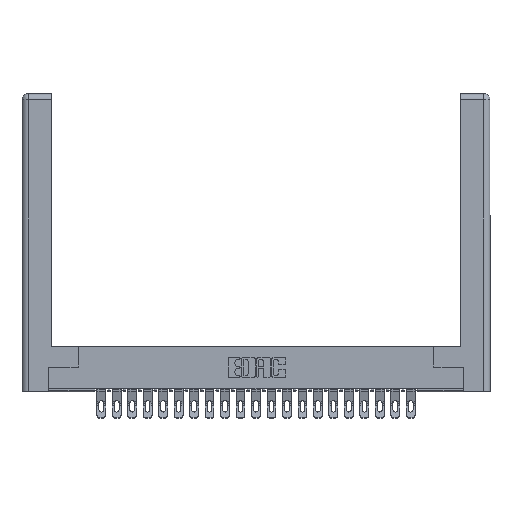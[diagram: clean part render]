
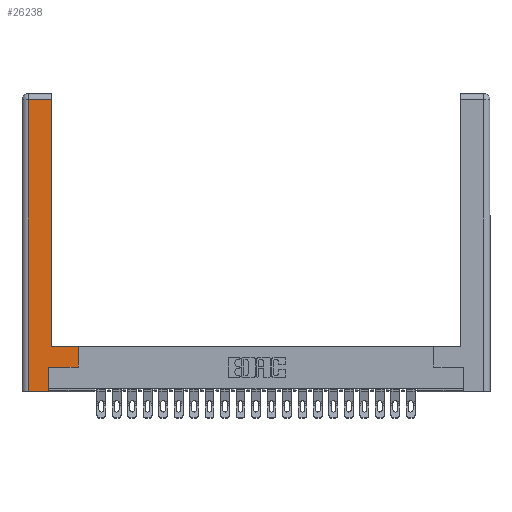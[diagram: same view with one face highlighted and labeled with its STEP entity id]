
A CAD part, top view. The second image highlights one B-rep face of the part: STEP entity #26238.
In plain terms, the highlighted planar face has unit normal (0, 0, 1).
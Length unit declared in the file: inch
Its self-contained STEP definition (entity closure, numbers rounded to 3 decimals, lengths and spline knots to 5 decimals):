
#41 = DIRECTION ( 'NONE',  ( 1., 0., 0. ) ) ;
#401 = VECTOR ( 'NONE', #19597, 39.37008 ) ;
#650 = CARTESIAN_POINT ( 'NONE',  ( 0.295, 3., 0. ) ) ;
#1685 = VERTEX_POINT ( 'NONE', #19593 ) ;
#1718 = EDGE_CURVE ( 'NONE', #11943, #3793, #8278, .T. ) ;
#2251 = LINE ( 'NONE', #16397, #21236 ) ;
#2384 = CARTESIAN_POINT ( 'NONE',  ( 0.295, 0.45, 0. ) ) ;
#2505 = LINE ( 'NONE', #15176, #26287 ) ;
#2629 = CARTESIAN_POINT ( 'NONE',  ( 0.565, 0.245, 0. ) ) ;
#2864 = ORIENTED_EDGE ( 'NONE', *, *, #25627, .T. ) ;
#3481 = ORIENTED_EDGE ( 'NONE', *, *, #10240, .T. ) ;
#3599 = VERTEX_POINT ( 'NONE', #26825 ) ;
#3793 = VERTEX_POINT ( 'NONE', #23927 ) ;
#4096 = CARTESIAN_POINT ( 'NONE',  ( 0.265, 0.245, 0. ) ) ;
#4238 = PLANE ( 'NONE',  #27831 ) ;
#4400 = VECTOR ( 'NONE', #17671, 39.37008 ) ;
#5527 = EDGE_CURVE ( 'NONE', #20513, #26955, #21147, .T. ) ;
#5560 = VERTEX_POINT ( 'NONE', #6835 ) ;
#5890 = ORIENTED_EDGE ( 'NONE', *, *, #1718, .T. ) ;
#6835 = CARTESIAN_POINT ( 'NONE',  ( 0.0615, 0., 0. ) ) ;
#7512 = LINE ( 'NONE', #8667, #4400 ) ;
#7633 = ORIENTED_EDGE ( 'NONE', *, *, #18144, .T. ) ;
#8278 = LINE ( 'NONE', #4096, #25208 ) ;
#8667 = CARTESIAN_POINT ( 'NONE',  ( 0.0615, 2.94, 0. ) ) ;
#10240 = EDGE_CURVE ( 'NONE', #1685, #3599, #21048, .T. ) ;
#10799 = DIRECTION ( 'NONE',  ( 0., 1., 0. ) ) ;
#10915 = ORIENTED_EDGE ( 'NONE', *, *, #24230, .T. ) ;
#11812 = DIRECTION ( 'NONE',  ( 0., 0., -1. ) ) ;
#11943 = VERTEX_POINT ( 'NONE', #23610 ) ;
#12116 = CARTESIAN_POINT ( 'NONE',  ( 0.0615, 0., 0. ) ) ;
#12366 = FACE_OUTER_BOUND ( 'NONE', #16614, .T. ) ;
#13110 = DIRECTION ( 'NONE',  ( -1., 0., 0. ) ) ;
#13130 = VECTOR ( 'NONE', #24866, 39.37008 ) ;
#13719 = VECTOR ( 'NONE', #13110, 39.37008 ) ;
#15030 = ORIENTED_EDGE ( 'NONE', *, *, #5527, .T. ) ;
#15176 = CARTESIAN_POINT ( 'NONE',  ( 0.265, 0., 0. ) ) ;
#16397 = CARTESIAN_POINT ( 'NONE',  ( 0.565, 0.245, 0. ) ) ;
#16427 = DIRECTION ( 'NONE',  ( -1., 0., 0. ) ) ;
#16614 = EDGE_LOOP ( 'NONE', ( #3481, #2864, #10915, #28482, #5890, #17641, #15030, #7633 ) ) ;
#17641 = ORIENTED_EDGE ( 'NONE', *, *, #18723, .T. ) ;
#17671 = DIRECTION ( 'NONE',  ( -1., 0., 0. ) ) ;
#18144 = EDGE_CURVE ( 'NONE', #26955, #1685, #25396, .T. ) ;
#18723 = EDGE_CURVE ( 'NONE', #3793, #20513, #2251, .T. ) ;
#18826 = DIRECTION ( 'NONE',  ( 1., 0., 0. ) ) ;
#19593 = CARTESIAN_POINT ( 'NONE',  ( 0.295, 0.45, 0. ) ) ;
#19597 = DIRECTION ( 'NONE',  ( 0., -1., 0. ) ) ;
#20261 = CARTESIAN_POINT ( 'NONE',  ( 0.0615, 2.94, 0. ) ) ;
#20348 = EDGE_CURVE ( 'NONE', #5560, #11943, #2505, .T. ) ;
#20513 = VERTEX_POINT ( 'NONE', #2629 ) ;
#20572 = CARTESIAN_POINT ( 'NONE',  ( 0., 0., 0. ) ) ;
#21048 = LINE ( 'NONE', #650, #13130 ) ;
#21147 = LINE ( 'NONE', #24435, #22527 ) ;
#21236 = VECTOR ( 'NONE', #18826, 39.37008 ) ;
#21810 = CARTESIAN_POINT ( 'NONE',  ( 0.565, 0.45, 0. ) ) ;
#22475 = LINE ( 'NONE', #12116, #401 ) ;
#22527 = VECTOR ( 'NONE', #26642, 39.37008 ) ;
#23103 = VERTEX_POINT ( 'NONE', #20261 ) ;
#23610 = CARTESIAN_POINT ( 'NONE',  ( 0.265, 0., 0. ) ) ;
#23927 = CARTESIAN_POINT ( 'NONE',  ( 0.265, 0.245, 0. ) ) ;
#24230 = EDGE_CURVE ( 'NONE', #23103, #5560, #22475, .T. ) ;
#24435 = CARTESIAN_POINT ( 'NONE',  ( 0.565, 0.45, 0. ) ) ;
#24866 = DIRECTION ( 'NONE',  ( 0., 1., 0. ) ) ;
#25208 = VECTOR ( 'NONE', #10799, 39.37008 ) ;
#25396 = LINE ( 'NONE', #2384, #13719 ) ;
#25627 = EDGE_CURVE ( 'NONE', #3599, #23103, #7512, .T. ) ;
#26238 = ADVANCED_FACE ( 'NONE', ( #12366 ), #4238, .F. ) ;
#26287 = VECTOR ( 'NONE', #41, 39.37008 ) ;
#26642 = DIRECTION ( 'NONE',  ( 0., 1., 0. ) ) ;
#26825 = CARTESIAN_POINT ( 'NONE',  ( 0.295, 2.94, 0. ) ) ;
#26955 = VERTEX_POINT ( 'NONE', #21810 ) ;
#27831 = AXIS2_PLACEMENT_3D ( 'NONE', #20572, #11812, #16427 ) ;
#28482 = ORIENTED_EDGE ( 'NONE', *, *, #20348, .T. ) ;
